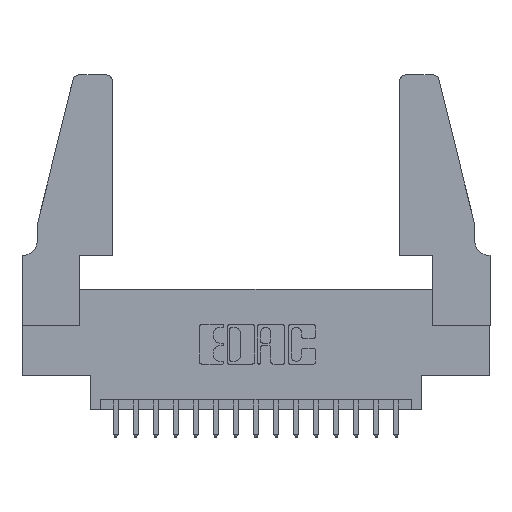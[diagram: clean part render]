
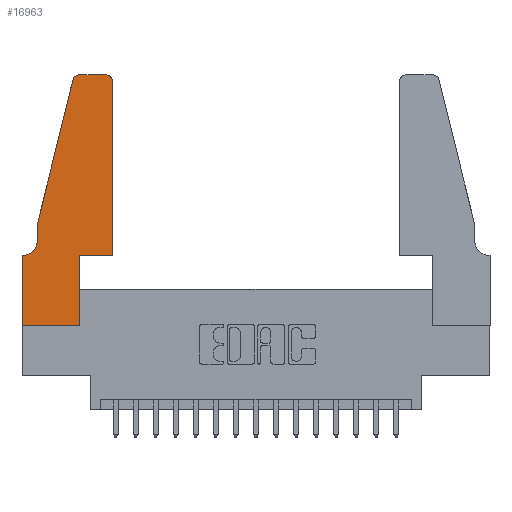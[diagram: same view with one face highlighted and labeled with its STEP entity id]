
A CAD part, top view. The second image highlights one B-rep face of the part: STEP entity #16963.
In plain terms, the highlighted planar face has unit normal (0, 0, 1).
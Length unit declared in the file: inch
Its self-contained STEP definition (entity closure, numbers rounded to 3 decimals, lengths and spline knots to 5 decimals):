
#333 = DIRECTION ( 'NONE',  ( -1., 0., 0. ) ) ;
#386 = CARTESIAN_POINT ( 'NONE',  ( 0.2865, 0., 0.37 ) ) ;
#427 = CARTESIAN_POINT ( 'NONE',  ( 0., 0., 0.37 ) ) ;
#556 = CIRCLE ( 'NONE', #1389, 0.07 ) ;
#567 = CARTESIAN_POINT ( 'NONE',  ( 0., 0.35, 0.37 ) ) ;
#614 = EDGE_CURVE ( 'NONE', #4507, #10845, #556, .T. ) ;
#1206 = ORIENTED_EDGE ( 'NONE', *, *, #12048, .T. ) ;
#1337 = EDGE_CURVE ( 'NONE', #3852, #4507, #6957, .T. ) ;
#1389 = AXIS2_PLACEMENT_3D ( 'NONE', #7147, #8507, #333 ) ;
#1411 = VECTOR ( 'NONE', #9726, 39.37008 ) ;
#1614 = CARTESIAN_POINT ( 'NONE',  ( 0.0755, 0.5, 0.37 ) ) ;
#1635 = EDGE_CURVE ( 'NONE', #13941, #6156, #16146, .T. ) ;
#1648 = VECTOR ( 'NONE', #8842, 39.37008 ) ;
#2384 = ORIENTED_EDGE ( 'NONE', *, *, #10394, .T. ) ;
#3617 = DIRECTION ( 'NONE',  ( 0., 0., 1. ) ) ;
#3776 = DIRECTION ( 'NONE',  ( -1., 0., 0. ) ) ;
#3852 = VERTEX_POINT ( 'NONE', #3883 ) ;
#3883 = CARTESIAN_POINT ( 'NONE',  ( 0.0755, 0.5, 0.37 ) ) ;
#3916 = ORIENTED_EDGE ( 'NONE', *, *, #6523, .T. ) ;
#3923 = AXIS2_PLACEMENT_3D ( 'NONE', #6917, #15056, #6859 ) ;
#4117 = CARTESIAN_POINT ( 'NONE',  ( 0.4205, 1.22, 0.37 ) ) ;
#4260 = LINE ( 'NONE', #6131, #1648 ) ;
#4507 = VERTEX_POINT ( 'NONE', #6312 ) ;
#4546 = VECTOR ( 'NONE', #3776, 39.37008 ) ;
#4630 = ORIENTED_EDGE ( 'NONE', *, *, #13031, .T. ) ;
#5422 = CARTESIAN_POINT ( 'NONE',  ( 0., 0., 0.37 ) ) ;
#5494 = DIRECTION ( 'NONE',  ( 1., 0., 0. ) ) ;
#5506 = PLANE ( 'NONE',  #3923 ) ;
#5578 = CARTESIAN_POINT ( 'NONE',  ( 0.0755, 0.5, 0.37 ) ) ;
#5602 = VERTEX_POINT ( 'NONE', #386 ) ;
#5994 = EDGE_CURVE ( 'NONE', #15266, #13941, #13500, .T. ) ;
#6131 = CARTESIAN_POINT ( 'NONE',  ( 0.4505, 0.35, 0.37 ) ) ;
#6156 = VERTEX_POINT ( 'NONE', #17367 ) ;
#6312 = CARTESIAN_POINT ( 'NONE',  ( 0.0755, 0.42, 0.37 ) ) ;
#6453 = CARTESIAN_POINT ( 'NONE',  ( 0.2865, 0.35, 0.37 ) ) ;
#6523 = EDGE_CURVE ( 'NONE', #9066, #9597, #7431, .T. ) ;
#6687 = DIRECTION ( 'NONE',  ( 1., 0., 0. ) ) ;
#6859 = DIRECTION ( 'NONE',  ( 1., 0., 0. ) ) ;
#6917 = CARTESIAN_POINT ( 'NONE',  ( 0., 0.35, 0.37 ) ) ;
#6957 = LINE ( 'NONE', #5578, #17451 ) ;
#7057 = ORIENTED_EDGE ( 'NONE', *, *, #5994, .T. ) ;
#7147 = CARTESIAN_POINT ( 'NONE',  ( 0.0055, 0.42, 0.37 ) ) ;
#7369 = ORIENTED_EDGE ( 'NONE', *, *, #14621, .T. ) ;
#7375 = LINE ( 'NONE', #12222, #1411 ) ;
#7418 = FACE_OUTER_BOUND ( 'NONE', #8552, .T. ) ;
#7431 = CIRCLE ( 'NONE', #12106, 0.03 ) ;
#7565 = VECTOR ( 'NONE', #11205, 39.37008 ) ;
#7655 = CARTESIAN_POINT ( 'NONE',  ( 0.284, 1.22, 0.37 ) ) ;
#7786 = DIRECTION ( 'NONE',  ( 1., 0., 0. ) ) ;
#8071 = ORIENTED_EDGE ( 'NONE', *, *, #1337, .T. ) ;
#8504 = CARTESIAN_POINT ( 'NONE',  ( 0.4505, 0.35, 0.37 ) ) ;
#8507 = DIRECTION ( 'NONE',  ( 0., 0., -1. ) ) ;
#8552 = EDGE_LOOP ( 'NONE', ( #8597, #3916, #11892, #8071, #11741, #16145, #1206, #4630, #2384, #7369, #7057, #10081 ) ) ;
#8597 = ORIENTED_EDGE ( 'NONE', *, *, #10853, .T. ) ;
#8732 = VECTOR ( 'NONE', #11330, 39.37008 ) ;
#8842 = DIRECTION ( 'NONE',  ( 1., 0., 0. ) ) ;
#8847 = LINE ( 'NONE', #427, #7565 ) ;
#9066 = VERTEX_POINT ( 'NONE', #14926 ) ;
#9597 = VERTEX_POINT ( 'NONE', #12436 ) ;
#9726 = DIRECTION ( 'NONE',  ( -1., 0., 0. ) ) ;
#9839 = DIRECTION ( 'NONE',  ( -0.239, -0.971, 0. ) ) ;
#10081 = ORIENTED_EDGE ( 'NONE', *, *, #1635, .T. ) ;
#10167 = LINE ( 'NONE', #13126, #16603 ) ;
#10357 = DIRECTION ( 'NONE',  ( 0., 1., 0. ) ) ;
#10394 = EDGE_CURVE ( 'NONE', #5602, #16789, #10167, .T. ) ;
#10845 = VERTEX_POINT ( 'NONE', #13951 ) ;
#10853 = EDGE_CURVE ( 'NONE', #6156, #9066, #7375, .T. ) ;
#10856 = EDGE_CURVE ( 'NONE', #9597, #3852, #17452, .T. ) ;
#11205 = DIRECTION ( 'NONE',  ( 0., -1., 0. ) ) ;
#11292 = CARTESIAN_POINT ( 'NONE',  ( 0.4505, 1.22, 0.37 ) ) ;
#11330 = DIRECTION ( 'NONE',  ( 0., 1., 0. ) ) ;
#11741 = ORIENTED_EDGE ( 'NONE', *, *, #614, .T. ) ;
#11797 = LINE ( 'NONE', #16094, #4546 ) ;
#11892 = ORIENTED_EDGE ( 'NONE', *, *, #10856, .T. ) ;
#12048 = EDGE_CURVE ( 'NONE', #14963, #17601, #8847, .T. ) ;
#12106 = AXIS2_PLACEMENT_3D ( 'NONE', #7655, #3617, #7786 ) ;
#12222 = CARTESIAN_POINT ( 'NONE',  ( 0.2605, 1.25, 0.37 ) ) ;
#12436 = CARTESIAN_POINT ( 'NONE',  ( 0.25487, 1.22718, 0.37 ) ) ;
#12899 = VECTOR ( 'NONE', #6687, 39.37008 ) ;
#13031 = EDGE_CURVE ( 'NONE', #17601, #5602, #15030, .T. ) ;
#13126 = CARTESIAN_POINT ( 'NONE',  ( 0.2865, 0.35, 0.37 ) ) ;
#13447 = DIRECTION ( 'NONE',  ( 0., 0., 1. ) ) ;
#13500 = LINE ( 'NONE', #8504, #8732 ) ;
#13521 = CARTESIAN_POINT ( 'NONE',  ( 0., 0., 0.37 ) ) ;
#13639 = EDGE_CURVE ( 'NONE', #10845, #14963, #11797, .T. ) ;
#13821 = VECTOR ( 'NONE', #9839, 39.37008 ) ;
#13941 = VERTEX_POINT ( 'NONE', #11292 ) ;
#13951 = CARTESIAN_POINT ( 'NONE',  ( 0.0055, 0.35, 0.37 ) ) ;
#14621 = EDGE_CURVE ( 'NONE', #16789, #15266, #4260, .T. ) ;
#14926 = CARTESIAN_POINT ( 'NONE',  ( 0.284, 1.25, 0.37 ) ) ;
#14963 = VERTEX_POINT ( 'NONE', #567 ) ;
#14976 = CARTESIAN_POINT ( 'NONE',  ( 0.4505, 0.35, 0.37 ) ) ;
#15030 = LINE ( 'NONE', #13521, #12899 ) ;
#15056 = DIRECTION ( 'NONE',  ( 0., 0., 1. ) ) ;
#15134 = DIRECTION ( 'NONE',  ( 0., -1., 0. ) ) ;
#15266 = VERTEX_POINT ( 'NONE', #14976 ) ;
#16094 = CARTESIAN_POINT ( 'NONE',  ( 0.0755, 0.35, 0.37 ) ) ;
#16145 = ORIENTED_EDGE ( 'NONE', *, *, #13639, .T. ) ;
#16146 = CIRCLE ( 'NONE', #16520, 0.03 ) ;
#16520 = AXIS2_PLACEMENT_3D ( 'NONE', #4117, #13447, #5494 ) ;
#16603 = VECTOR ( 'NONE', #10357, 39.37008 ) ;
#16789 = VERTEX_POINT ( 'NONE', #6453 ) ;
#16963 = ADVANCED_FACE ( 'NONE', ( #7418 ), #5506, .T. ) ;
#17367 = CARTESIAN_POINT ( 'NONE',  ( 0.4205, 1.25, 0.37 ) ) ;
#17451 = VECTOR ( 'NONE', #15134, 39.37008 ) ;
#17452 = LINE ( 'NONE', #1614, #13821 ) ;
#17601 = VERTEX_POINT ( 'NONE', #5422 ) ;
